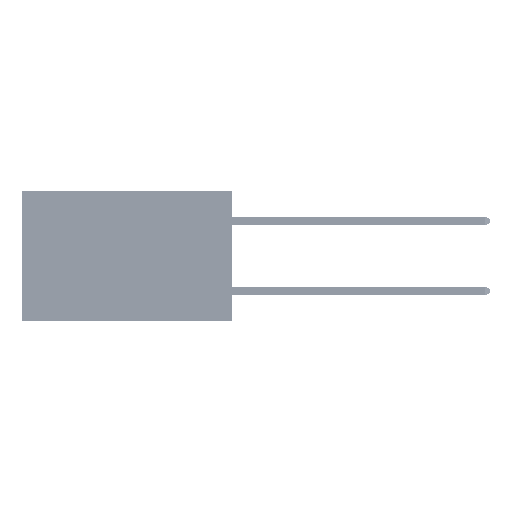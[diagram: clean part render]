
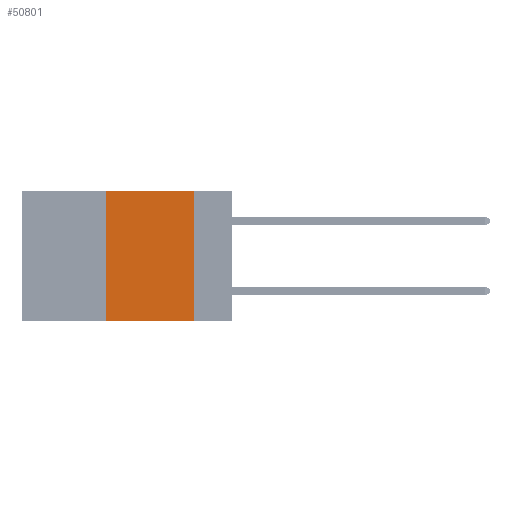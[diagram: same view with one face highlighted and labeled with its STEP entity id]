
A CAD part, left-side view. The second image highlights one B-rep face of the part: STEP entity #50801.
In plain terms, the highlighted planar face has unit normal (-1, 0, 0).
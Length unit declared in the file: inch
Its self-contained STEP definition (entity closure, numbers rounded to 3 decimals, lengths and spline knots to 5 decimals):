
#385 = EDGE_CURVE ( 'NONE', #33855, #23067, #14454, .T. ) ;
#406 = CARTESIAN_POINT ( 'NONE',  ( 0., 0.36, 0. ) ) ;
#813 = CARTESIAN_POINT ( 'NONE',  ( 0., 0.6, 0. ) ) ;
#1300 = AXIS2_PLACEMENT_3D ( 'NONE', #8794, #4771, #35784 ) ;
#2203 = VERTEX_POINT ( 'NONE', #38875 ) ;
#2571 = VECTOR ( 'NONE', #43770, 39.37008 ) ;
#3239 = CARTESIAN_POINT ( 'NONE',  ( 0., 0.6, -0.37 ) ) ;
#3900 = VECTOR ( 'NONE', #33426, 39.37008 ) ;
#4192 = VECTOR ( 'NONE', #21236, 39.37008 ) ;
#4771 = DIRECTION ( 'NONE',  ( 1., 0., 0. ) ) ;
#5700 = LINE ( 'NONE', #16090, #2571 ) ;
#6837 = CARTESIAN_POINT ( 'NONE',  ( 0., 0.11, 0. ) ) ;
#7229 = EDGE_CURVE ( 'NONE', #23067, #42389, #40970, .T. ) ;
#8032 = ORIENTED_EDGE ( 'NONE', *, *, #14005, .F. ) ;
#8794 = CARTESIAN_POINT ( 'NONE',  ( 0., 0.6, 0. ) ) ;
#9977 = ORIENTED_EDGE ( 'NONE', *, *, #385, .F. ) ;
#14005 = EDGE_CURVE ( 'NONE', #42389, #2203, #5700, .T. ) ;
#14454 = LINE ( 'NONE', #37718, #3900 ) ;
#16090 = CARTESIAN_POINT ( 'NONE',  ( 0., 0.11, 0. ) ) ;
#17756 = LINE ( 'NONE', #3239, #38225 ) ;
#17920 = ORIENTED_EDGE ( 'NONE', *, *, #25054, .T. ) ;
#20239 = FACE_OUTER_BOUND ( 'NONE', #40633, .T. ) ;
#21236 = DIRECTION ( 'NONE',  ( 0., -1., 0. ) ) ;
#23067 = VERTEX_POINT ( 'NONE', #406 ) ;
#25054 = EDGE_CURVE ( 'NONE', #33855, #2203, #17756, .T. ) ;
#32336 = PLANE ( 'NONE',  #1300 ) ;
#33426 = DIRECTION ( 'NONE',  ( 0., 0., 1. ) ) ;
#33855 = VERTEX_POINT ( 'NONE', #36163 ) ;
#35784 = DIRECTION ( 'NONE',  ( 0., 0., -1. ) ) ;
#36163 = CARTESIAN_POINT ( 'NONE',  ( 0., 0.36, -0.37 ) ) ;
#37718 = CARTESIAN_POINT ( 'NONE',  ( 0., 0.36, 0. ) ) ;
#38225 = VECTOR ( 'NONE', #46488, 39.37008 ) ;
#38875 = CARTESIAN_POINT ( 'NONE',  ( 0., 0.11, -0.37 ) ) ;
#40633 = EDGE_LOOP ( 'NONE', ( #8032, #43276, #9977, #17920 ) ) ;
#40970 = LINE ( 'NONE', #813, #4192 ) ;
#42389 = VERTEX_POINT ( 'NONE', #6837 ) ;
#43276 = ORIENTED_EDGE ( 'NONE', *, *, #7229, .F. ) ;
#43770 = DIRECTION ( 'NONE',  ( 0., 0., -1. ) ) ;
#46488 = DIRECTION ( 'NONE',  ( 0., -1., 0. ) ) ;
#50801 = ADVANCED_FACE ( 'NONE', ( #20239 ), #32336, .F. ) ;
